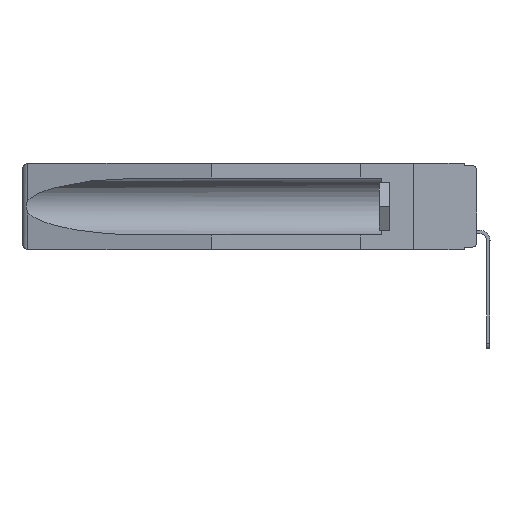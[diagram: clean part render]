
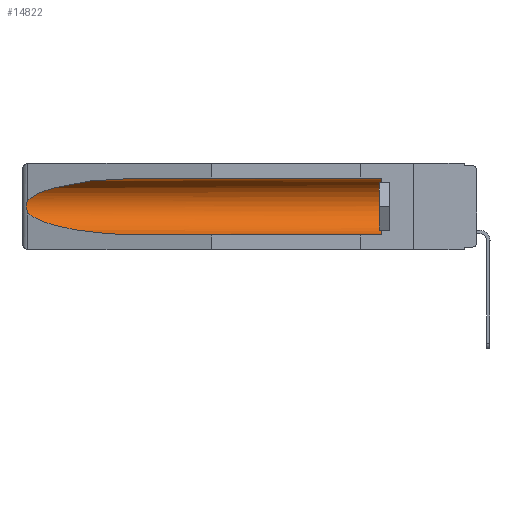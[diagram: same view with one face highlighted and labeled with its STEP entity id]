
A CAD part, left-side view. The second image highlights one B-rep face of the part: STEP entity #14822.
In plain terms, the highlighted cylindrical face has radius 2.857 mm (diameter 5.715 mm), a partial arc.
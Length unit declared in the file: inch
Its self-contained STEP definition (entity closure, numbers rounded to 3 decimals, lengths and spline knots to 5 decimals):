
#83 = CARTESIAN_POINT ( 'NONE',  ( 0.2673, 1.5327, -0.16383 ) ) ;
#145 = EDGE_CURVE ( 'NONE', #15944, #11403, #451, .T. ) ;
#451 = B_SPLINE_CURVE_WITH_KNOTS ( 'NONE', 3,
 ( #11740, #4106, #7723, #83, #13403, #7800, #5324, #13143, #10607, #15948 ),
 .UNSPECIFIED., .F., .F.,
 ( 4, 2, 2, 2, 4 ),
 ( 0., 0.00029, 0.00058, 0.00087, 0.00117 ),
 .UNSPECIFIED. ) ;
#632 = CARTESIAN_POINT ( 'NONE',  ( 0.155, -0.30754, -0.1715 ) ) ;
#730 = LINE ( 'NONE', #11426, #15980 ) ;
#1217 = CIRCLE ( 'NONE', #15774, 0.1125 ) ;
#1289 = CARTESIAN_POINT ( 'NONE',  ( 0.26537, 1.52718, -0.19328 ) ) ;
#1769 = DIRECTION ( 'NONE',  ( 0., 1., 0. ) ) ;
#1851 = DIRECTION ( 'NONE',  ( 0., 0., 1. ) ) ;
#2079 = ORIENTED_EDGE ( 'NONE', *, *, #8740, .T. ) ;
#2195 = EDGE_CURVE ( 'NONE', #11403, #15425, #14756, .T. ) ;
#2328 = CARTESIAN_POINT ( 'NONE',  ( 0.155, 1.07973, -0.284 ) ) ;
#2573 = CARTESIAN_POINT ( 'NONE',  ( 0.155, 1.07973, -0.059 ) ) ;
#3050 = ORIENTED_EDGE ( 'NONE', *, *, #2195, .T. ) ;
#3247 = DIRECTION ( 'NONE',  ( 0., 1., 0. ) ) ;
#3335 = LINE ( 'NONE', #16559, #9002 ) ;
#4106 = CARTESIAN_POINT ( 'NONE',  ( 0.26597, 1.52961, -0.15275 ) ) ;
#4166 = AXIS2_PLACEMENT_3D ( 'NONE', #632, #1769, #1851 ) ;
#4222 = EDGE_CURVE ( 'NONE', #5107, #7454, #730, .T. ) ;
#4457 = EDGE_CURVE ( 'NONE', #5953, #15425, #3335, .T. ) ;
#4800 = DIRECTION ( 'NONE',  ( 0., 0., 1. ) ) ;
#5107 = VERTEX_POINT ( 'NONE', #15340 ) ;
#5324 = CARTESIAN_POINT ( 'NONE',  ( 0.2673, 1.53269, -0.17917 ) ) ;
#5649 = ORIENTED_EDGE ( 'NONE', *, *, #11366, .T. ) ;
#5797 = CARTESIAN_POINT ( 'NONE',  ( 0.26537, 1.52718, -0.14972 ) ) ;
#5946 = DIRECTION ( 'NONE',  ( 0., -1., 0. ) ) ;
#5953 = VERTEX_POINT ( 'NONE', #6890 ) ;
#6851 = ORIENTED_EDGE ( 'NONE', *, *, #145, .T. ) ;
#6890 = CARTESIAN_POINT ( 'NONE',  ( 0.155, 0.126, -0.284 ) ) ;
#7294 = FACE_OUTER_BOUND ( 'NONE', #13121, .T. ) ;
#7454 = VERTEX_POINT ( 'NONE', #2573 ) ;
#7723 = CARTESIAN_POINT ( 'NONE',  ( 0.26654, 1.53092, -0.15636 ) ) ;
#7800 = CARTESIAN_POINT ( 'NONE',  ( 0.2675, 1.53308, -0.17534 ) ) ;
#8740 = EDGE_CURVE ( 'NONE', #5953, #5107, #1217, .T. ) ;
#8932 = CARTESIAN_POINT ( 'NONE',  ( 0.155, 0.126, -0.1715 ) ) ;
#9002 = VECTOR ( 'NONE', #3247, 39.37008 ) ;
#10295 = ORIENTED_EDGE ( 'NONE', *, *, #4222, .T. ) ;
#10328 = CARTESIAN_POINT ( 'NONE',  ( 0.155, 1.07973, -0.284 ) ) ;
#10498 = CARTESIAN_POINT ( 'NONE',  ( 0.26537, 1.52718, -0.19328 ) ) ;
#10607 = CARTESIAN_POINT ( 'NONE',  ( 0.26597, 1.5296, -0.19026 ) ) ;
#10681 = ORIENTED_EDGE ( 'NONE', *, *, #4457, .F. ) ;
#10807 = CARTESIAN_POINT ( 'NONE',  ( 0.26537, 1.52718, -0.14972 ) ) ;
#11366 = EDGE_CURVE ( 'NONE', #7454, #15944, #16567, .T. ) ;
#11403 = VERTEX_POINT ( 'NONE', #1289 ) ;
#11426 = CARTESIAN_POINT ( 'NONE',  ( 0.155, -0.30754, -0.059 ) ) ;
#11740 = CARTESIAN_POINT ( 'NONE',  ( 0.26537, 1.52718, -0.14972 ) ) ;
#11796 = CARTESIAN_POINT ( 'NONE',  ( 0.21114, 1.30732, -0.284 ) ) ;
#11882 = CARTESIAN_POINT ( 'NONE',  ( 0.25451, 1.48313, -0.24835 ) ) ;
#12642 = CYLINDRICAL_SURFACE ( 'NONE', #4166, 0.1125 ) ;
#13121 = EDGE_LOOP ( 'NONE', ( #5649, #6851, #3050, #10681, #2079, #10295 ) ) ;
#13143 = CARTESIAN_POINT ( 'NONE',  ( 0.26655, 1.53094, -0.18657 ) ) ;
#13403 = CARTESIAN_POINT ( 'NONE',  ( 0.2675, 1.53308, -0.16763 ) ) ;
#13780 = CARTESIAN_POINT ( 'NONE',  ( 0.25451, 1.48313, -0.09465 ) ) ;
#14756 =( BOUNDED_CURVE ( )  B_SPLINE_CURVE ( 3, ( #10498, #11882, #11796, #10328 ),
 .UNSPECIFIED., .F., .F. ) 
 B_SPLINE_CURVE_WITH_KNOTS ( ( 4, 4 ),
 ( 0.1948, 1.5708 ),
 .UNSPECIFIED. ) 
 CURVE ( )  GEOMETRIC_REPRESENTATION_ITEM ( )  RATIONAL_B_SPLINE_CURVE ( ( 1., 0.848, 0.848, 1. ) ) 
 REPRESENTATION_ITEM ( '' )  );
#14822 = ADVANCED_FACE ( 'NONE', ( #7294 ), #12642, .F. ) ;
#15181 = CARTESIAN_POINT ( 'NONE',  ( 0.21114, 1.30732, -0.059 ) ) ;
#15340 = CARTESIAN_POINT ( 'NONE',  ( 0.155, 0.126, -0.059 ) ) ;
#15425 = VERTEX_POINT ( 'NONE', #2328 ) ;
#15441 = CARTESIAN_POINT ( 'NONE',  ( 0.155, 1.07973, -0.059 ) ) ;
#15774 = AXIS2_PLACEMENT_3D ( 'NONE', #8932, #5946, #4800 ) ;
#15944 = VERTEX_POINT ( 'NONE', #10807 ) ;
#15948 = CARTESIAN_POINT ( 'NONE',  ( 0.26537, 1.52718, -0.19328 ) ) ;
#15980 = VECTOR ( 'NONE', #16760, 39.37008 ) ;
#16559 = CARTESIAN_POINT ( 'NONE',  ( 0.155, -0.30754, -0.284 ) ) ;
#16567 =( BOUNDED_CURVE ( )  B_SPLINE_CURVE ( 3, ( #15441, #15181, #13780, #5797 ),
 .UNSPECIFIED., .F., .T. ) 
 B_SPLINE_CURVE_WITH_KNOTS ( ( 4, 4 ),
 ( 4.71239, 6.08839 ),
 .UNSPECIFIED. ) 
 CURVE ( )  GEOMETRIC_REPRESENTATION_ITEM ( )  RATIONAL_B_SPLINE_CURVE ( ( 1., 0.848, 0.848, 1. ) ) 
 REPRESENTATION_ITEM ( '' )  );
#16760 = DIRECTION ( 'NONE',  ( 0., 1., 0. ) ) ;
